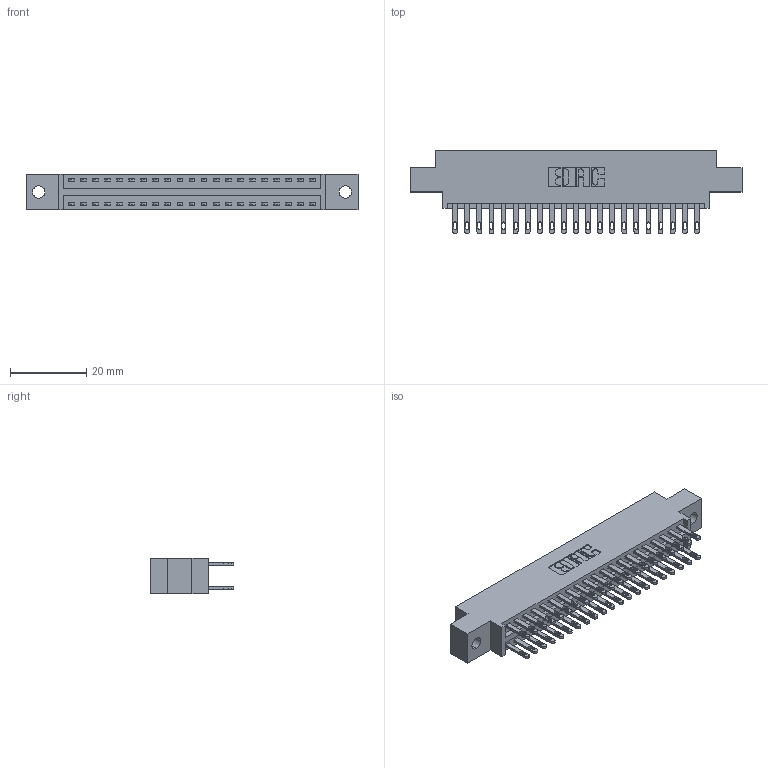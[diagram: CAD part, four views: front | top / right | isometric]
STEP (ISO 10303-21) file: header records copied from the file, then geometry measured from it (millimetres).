
FILE_DESCRIPTION (( 'STEP AP203' ), '1' );
FILE_NAME ('896-042-500-802.STEP', '2021-07-27T21:42:18', ( '' ), ( '' ), 'SwSTEP 2.0', 'SolidWorks 2020', '' );
FILE_SCHEMA (( 'CONFIG_CONTROL_DESIGN' ));
Length unit declared in the file: inch
Products named in the file (3): 896-042-500-802; 846 Part_0.170 Offset - 0.128 Dia; 345-292-001_345-293-100
Assembly tree (43 placements, depth 2):
  896-042-500-802
    846 Part_0.170 Offset - 0.128 Dia
    345-292-001_345-293-100  x42
Bounding box: 87.25 x 21.84 x 9.4 mm (x, y, z)
Volume: 8281.8 mm3; surface area: 11403.8 mm2
Topology: 43 solids, 43 shells, 2142 faces, 6515 edges, 4342 vertices
Faces by surface type: plane 1298, cylinder 844
Entity records: 16597 total; most frequent: CARTESIAN_POINT 2764, ORIENTED_EDGE 2698, DIRECTION 2489, EDGE_CURVE 1349, LINE 1129, VECTOR 1129, VERTEX_POINT 898, AXIS2_PLACEMENT_3D 680
